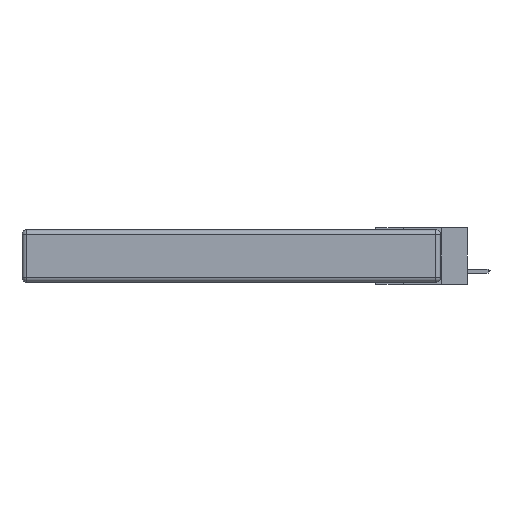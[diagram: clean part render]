
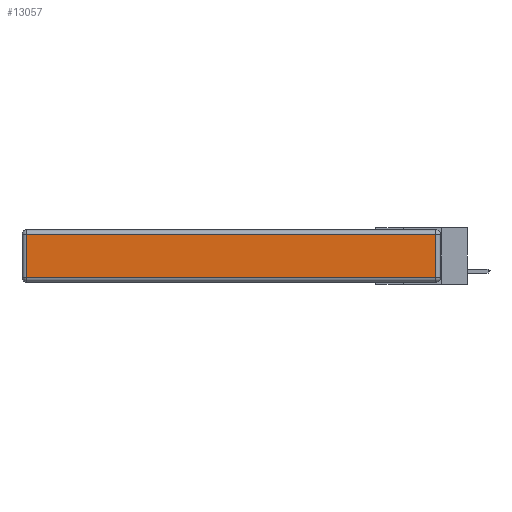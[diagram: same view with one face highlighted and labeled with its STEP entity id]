
A CAD part, left-side view. The second image highlights one B-rep face of the part: STEP entity #13057.
In plain terms, the highlighted planar face has unit normal (-1, 0, 0).
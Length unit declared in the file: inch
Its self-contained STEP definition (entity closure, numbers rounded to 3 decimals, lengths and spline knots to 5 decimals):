
#145 = VERTEX_POINT ( 'NONE', #9740 ) ;
#204 = LINE ( 'NONE', #7595, #10620 ) ;
#427 = DIRECTION ( 'NONE',  ( 0., 0., 1. ) ) ;
#816 = ORIENTED_EDGE ( 'NONE', *, *, #13720, .T. ) ;
#897 = ORIENTED_EDGE ( 'NONE', *, *, #2171, .T. ) ;
#1320 = CARTESIAN_POINT ( 'NONE',  ( 0., 0., -0.343 ) ) ;
#1338 = LINE ( 'NONE', #5059, #6352 ) ;
#1463 = VERTEX_POINT ( 'NONE', #4763 ) ;
#1753 = DIRECTION ( 'NONE',  ( 0., 0., 1. ) ) ;
#1760 = VERTEX_POINT ( 'NONE', #6624 ) ;
#2171 = EDGE_CURVE ( 'NONE', #1760, #1463, #12922, .T. ) ;
#2301 = EDGE_LOOP ( 'NONE', ( #816, #9317, #8736, #897 ) ) ;
#2317 = DIRECTION ( 'NONE',  ( 0., -1., 0. ) ) ;
#2845 = EDGE_CURVE ( 'NONE', #12172, #145, #1338, .T. ) ;
#3493 = CARTESIAN_POINT ( 'NONE',  ( 0., 0.03, -0.313 ) ) ;
#3660 = DIRECTION ( 'NONE',  ( 0., 0., -1. ) ) ;
#4602 = VECTOR ( 'NONE', #9436, 39.37008 ) ;
#4763 = CARTESIAN_POINT ( 'NONE',  ( 0., 2.72, -0.313 ) ) ;
#5059 = CARTESIAN_POINT ( 'NONE',  ( 0., 0.03, -0.343 ) ) ;
#6352 = VECTOR ( 'NONE', #1753, 39.37008 ) ;
#6624 = CARTESIAN_POINT ( 'NONE',  ( 0., 2.72, -0.03 ) ) ;
#7595 = CARTESIAN_POINT ( 'NONE',  ( 0., 0., -0.313 ) ) ;
#7691 = AXIS2_PLACEMENT_3D ( 'NONE', #1320, #9895, #427 ) ;
#7704 = VECTOR ( 'NONE', #3660, 39.37008 ) ;
#8736 = ORIENTED_EDGE ( 'NONE', *, *, #10942, .T. ) ;
#9317 = ORIENTED_EDGE ( 'NONE', *, *, #2845, .T. ) ;
#9436 = DIRECTION ( 'NONE',  ( 0., 1., 0. ) ) ;
#9740 = CARTESIAN_POINT ( 'NONE',  ( 0., 0.03, -0.03 ) ) ;
#9895 = DIRECTION ( 'NONE',  ( -1., 0., 0. ) ) ;
#10191 = LINE ( 'NONE', #10489, #4602 ) ;
#10489 = CARTESIAN_POINT ( 'NONE',  ( 0., 2.75, -0.03 ) ) ;
#10620 = VECTOR ( 'NONE', #2317, 39.37008 ) ;
#10942 = EDGE_CURVE ( 'NONE', #145, #1760, #10191, .T. ) ;
#11077 = CARTESIAN_POINT ( 'NONE',  ( 0., 2.72, -0.343 ) ) ;
#12172 = VERTEX_POINT ( 'NONE', #3493 ) ;
#12300 = FACE_OUTER_BOUND ( 'NONE', #2301, .T. ) ;
#12922 = LINE ( 'NONE', #11077, #7704 ) ;
#13057 = ADVANCED_FACE ( 'NONE', ( #12300 ), #13254, .T. ) ;
#13254 = PLANE ( 'NONE',  #7691 ) ;
#13720 = EDGE_CURVE ( 'NONE', #1463, #12172, #204, .T. ) ;
